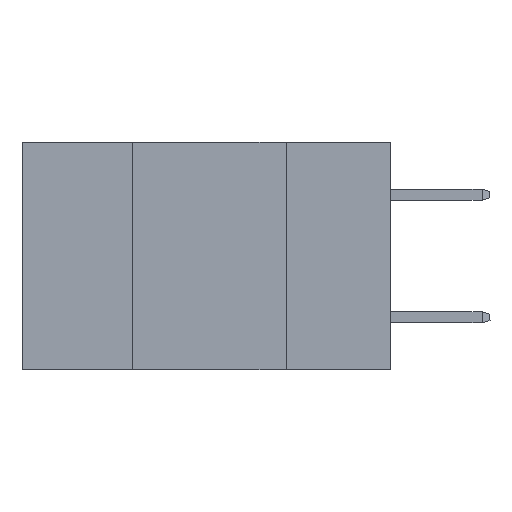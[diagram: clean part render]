
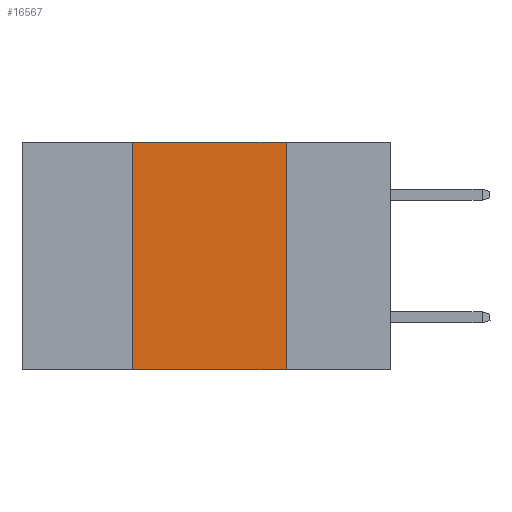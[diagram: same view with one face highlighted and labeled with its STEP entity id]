
A CAD part, left-side view. The second image highlights one B-rep face of the part: STEP entity #16567.
In plain terms, the highlighted planar face has unit normal (-1, 0, 0).
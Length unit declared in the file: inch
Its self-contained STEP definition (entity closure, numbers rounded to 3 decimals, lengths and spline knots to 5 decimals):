
#315 = DIRECTION ( 'NONE',  ( 1., 0., 0. ) ) ;
#707 = VECTOR ( 'NONE', #4878, 39.37008 ) ;
#1066 = EDGE_CURVE ( 'NONE', #9671, #11231, #8872, .T. ) ;
#1097 = LINE ( 'NONE', #11177, #8730 ) ;
#1101 = FACE_OUTER_BOUND ( 'NONE', #1955, .T. ) ;
#1756 = ORIENTED_EDGE ( 'NONE', *, *, #14366, .F. ) ;
#1955 = EDGE_LOOP ( 'NONE', ( #1756, #10991, #15022, #2153 ) ) ;
#2153 = ORIENTED_EDGE ( 'NONE', *, *, #6773, .T. ) ;
#3425 = CARTESIAN_POINT ( 'NONE',  ( 0., 0.17, 0. ) ) ;
#4878 = DIRECTION ( 'NONE',  ( 0., 0., 1. ) ) ;
#5213 = VECTOR ( 'NONE', #15355, 39.37008 ) ;
#6485 = VECTOR ( 'NONE', #11226, 39.37008 ) ;
#6773 = EDGE_CURVE ( 'NONE', #9671, #6793, #10494, .T. ) ;
#6793 = VERTEX_POINT ( 'NONE', #18813 ) ;
#7461 = CARTESIAN_POINT ( 'NONE',  ( 0., 0.42, 0. ) ) ;
#8730 = VECTOR ( 'NONE', #18499, 39.37008 ) ;
#8872 = LINE ( 'NONE', #7461, #707 ) ;
#9280 = LINE ( 'NONE', #3425, #5213 ) ;
#9512 = CARTESIAN_POINT ( 'NONE',  ( 0., 0.6, 0. ) ) ;
#9671 = VERTEX_POINT ( 'NONE', #18266 ) ;
#10348 = EDGE_CURVE ( 'NONE', #11231, #15240, #1097, .T. ) ;
#10494 = LINE ( 'NONE', #18481, #6485 ) ;
#10982 = DIRECTION ( 'NONE',  ( 0., 0., -1. ) ) ;
#10991 = ORIENTED_EDGE ( 'NONE', *, *, #10348, .F. ) ;
#11177 = CARTESIAN_POINT ( 'NONE',  ( 0., 0.6, 0. ) ) ;
#11226 = DIRECTION ( 'NONE',  ( 0., -1., 0. ) ) ;
#11231 = VERTEX_POINT ( 'NONE', #14553 ) ;
#12371 = PLANE ( 'NONE',  #13378 ) ;
#13378 = AXIS2_PLACEMENT_3D ( 'NONE', #9512, #315, #10982 ) ;
#14366 = EDGE_CURVE ( 'NONE', #15240, #6793, #9280, .T. ) ;
#14553 = CARTESIAN_POINT ( 'NONE',  ( 0., 0.42, 0. ) ) ;
#15022 = ORIENTED_EDGE ( 'NONE', *, *, #1066, .F. ) ;
#15240 = VERTEX_POINT ( 'NONE', #15248 ) ;
#15248 = CARTESIAN_POINT ( 'NONE',  ( 0., 0.17, 0. ) ) ;
#15355 = DIRECTION ( 'NONE',  ( 0., 0., -1. ) ) ;
#16567 = ADVANCED_FACE ( 'NONE', ( #1101 ), #12371, .F. ) ;
#18266 = CARTESIAN_POINT ( 'NONE',  ( 0., 0.42, -0.37 ) ) ;
#18481 = CARTESIAN_POINT ( 'NONE',  ( 0., 0.6, -0.37 ) ) ;
#18499 = DIRECTION ( 'NONE',  ( 0., -1., 0. ) ) ;
#18813 = CARTESIAN_POINT ( 'NONE',  ( 0., 0.17, -0.37 ) ) ;
